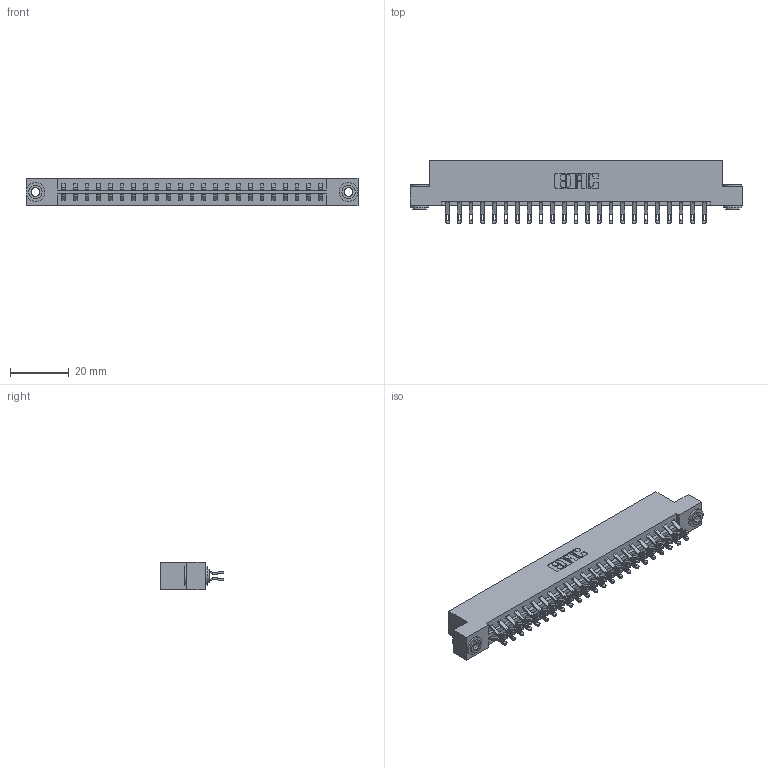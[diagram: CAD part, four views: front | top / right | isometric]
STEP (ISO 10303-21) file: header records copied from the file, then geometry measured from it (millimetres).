
FILE_DESCRIPTION (( 'STEP AP203' ), '1' );
FILE_NAME ('833-046-555-203.STEP', '2020-06-04T14:44:26', ( '' ), ( '' ), 'SwSTEP 2.0', 'SolidWorks 2020', '' );
FILE_SCHEMA (( 'CONFIG_CONTROL_DESIGN' ));
Length unit declared in the file: inch
Products named in the file (4): 833 Part_Flush - .156 Dia - TH; 345-292-001_555 Tail; 833-046-555-203; 345-250-002_345-250-002-102
Assembly tree (49 placements, depth 2):
  833-046-555-203
    833 Part_Flush - .156 Dia - TH
    345-292-001_555 Tail  x46
    345-250-002_345-250-002-102  x2
Bounding box: 112.67 x 21.47 x 9.4 mm (x, y, z)
Volume: 11478.5 mm3; surface area: 14086.2 mm2
Topology: 49 solids, 49 shells, 2820 faces, 8805 edges, 5866 vertices
Faces by surface type: plane 1644, cylinder 1168, cone 8
Entity records: 18230 total; most frequent: CARTESIAN_POINT 3055, ORIENTED_EDGE 2954, DIRECTION 2647, EDGE_CURVE 1477, LINE 1305, VECTOR 1305, VERTEX_POINT 982, AXIS2_PLACEMENT_3D 671
